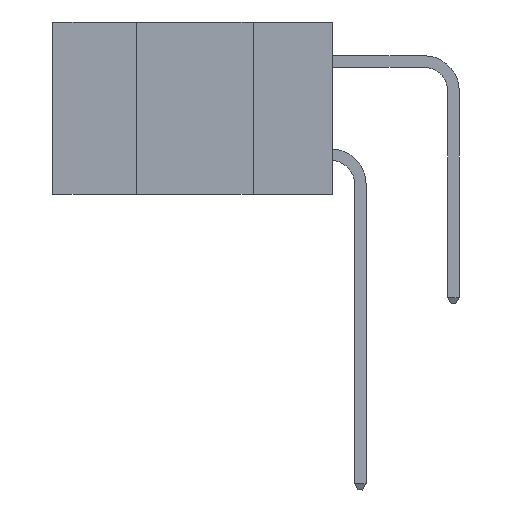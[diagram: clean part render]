
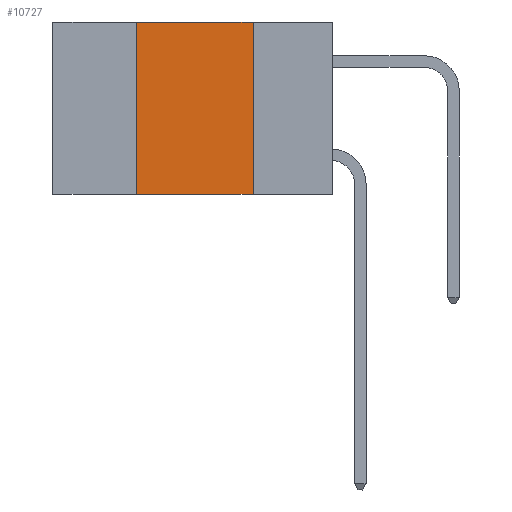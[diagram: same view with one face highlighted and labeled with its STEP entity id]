
A CAD part, left-side view. The second image highlights one B-rep face of the part: STEP entity #10727.
In plain terms, the highlighted planar face has unit normal (-1, 0, 0).
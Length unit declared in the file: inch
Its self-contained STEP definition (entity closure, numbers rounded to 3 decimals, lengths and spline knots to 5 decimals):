
#246 = EDGE_LOOP ( 'NONE', ( #1578, #1679, #1287, #2786 ) ) ;
#309 = PLANE ( 'NONE',  #3139 ) ;
#427 = VERTEX_POINT ( 'NONE', #7504 ) ;
#526 = LINE ( 'NONE', #4153, #2540 ) ;
#804 = DIRECTION ( 'NONE',  ( 0., 0., -1. ) ) ;
#813 = CARTESIAN_POINT ( 'NONE',  ( 0., 0.17, 0. ) ) ;
#822 = VECTOR ( 'NONE', #7022, 39.37008 ) ;
#1287 = ORIENTED_EDGE ( 'NONE', *, *, #10150, .F. ) ;
#1572 = FACE_OUTER_BOUND ( 'NONE', #246, .T. ) ;
#1578 = ORIENTED_EDGE ( 'NONE', *, *, #5009, .F. ) ;
#1583 = LINE ( 'NONE', #6762, #11118 ) ;
#1679 = ORIENTED_EDGE ( 'NONE', *, *, #2974, .F. ) ;
#1920 = VERTEX_POINT ( 'NONE', #10605 ) ;
#2540 = VECTOR ( 'NONE', #8188, 39.37008 ) ;
#2786 = ORIENTED_EDGE ( 'NONE', *, *, #9654, .T. ) ;
#2974 = EDGE_CURVE ( 'NONE', #4309, #1920, #526, .T. ) ;
#2987 = DIRECTION ( 'NONE',  ( 0., 0., -1. ) ) ;
#3139 = AXIS2_PLACEMENT_3D ( 'NONE', #5712, #8285, #2987 ) ;
#3174 = CARTESIAN_POINT ( 'NONE',  ( 0., 0.42, 0. ) ) ;
#3770 = LINE ( 'NONE', #813, #8462 ) ;
#4153 = CARTESIAN_POINT ( 'NONE',  ( 0., 0.6, 0. ) ) ;
#4309 = VERTEX_POINT ( 'NONE', #3174 ) ;
#5009 = EDGE_CURVE ( 'NONE', #1920, #10443, #3770, .T. ) ;
#5712 = CARTESIAN_POINT ( 'NONE',  ( 0., 0.6, 0. ) ) ;
#6242 = CARTESIAN_POINT ( 'NONE',  ( 0., 0.17, -0.37 ) ) ;
#6762 = CARTESIAN_POINT ( 'NONE',  ( 0., 0.42, 0. ) ) ;
#7022 = DIRECTION ( 'NONE',  ( 0., -1., 0. ) ) ;
#7504 = CARTESIAN_POINT ( 'NONE',  ( 0., 0.42, -0.37 ) ) ;
#7834 = CARTESIAN_POINT ( 'NONE',  ( 0., 0.6, -0.37 ) ) ;
#8137 = LINE ( 'NONE', #7834, #822 ) ;
#8188 = DIRECTION ( 'NONE',  ( 0., -1., 0. ) ) ;
#8285 = DIRECTION ( 'NONE',  ( 1., 0., 0. ) ) ;
#8462 = VECTOR ( 'NONE', #804, 39.37008 ) ;
#9317 = DIRECTION ( 'NONE',  ( 0., 0., 1. ) ) ;
#9654 = EDGE_CURVE ( 'NONE', #427, #10443, #8137, .T. ) ;
#10150 = EDGE_CURVE ( 'NONE', #427, #4309, #1583, .T. ) ;
#10443 = VERTEX_POINT ( 'NONE', #6242 ) ;
#10605 = CARTESIAN_POINT ( 'NONE',  ( 0., 0.17, 0. ) ) ;
#10727 = ADVANCED_FACE ( 'NONE', ( #1572 ), #309, .F. ) ;
#11118 = VECTOR ( 'NONE', #9317, 39.37008 ) ;
